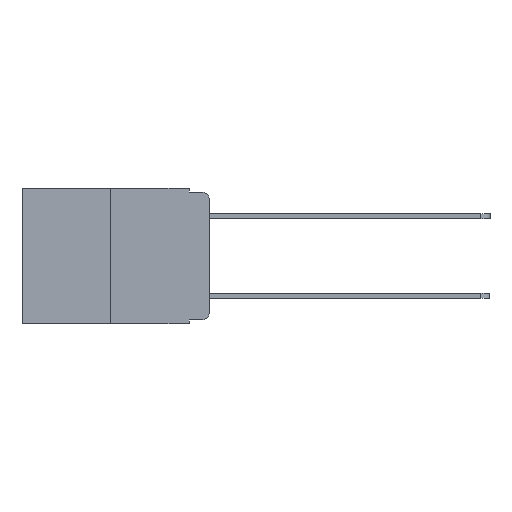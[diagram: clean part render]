
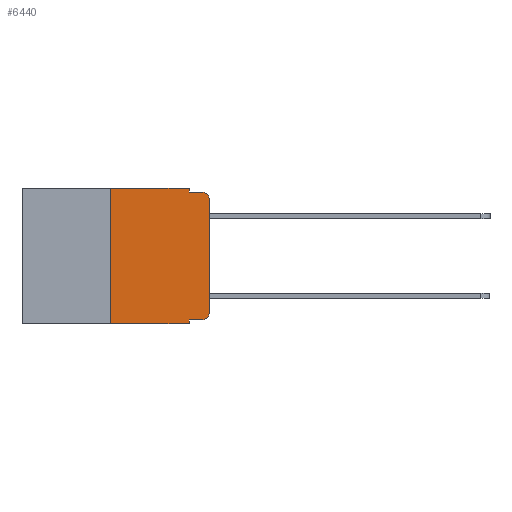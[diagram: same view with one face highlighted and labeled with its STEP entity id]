
A CAD part, left-side view. The second image highlights one B-rep face of the part: STEP entity #6440.
In plain terms, the highlighted planar face has unit normal (-1, 0, 0).
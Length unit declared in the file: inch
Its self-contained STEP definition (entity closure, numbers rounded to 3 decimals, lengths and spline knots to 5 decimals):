
#75 = VERTEX_POINT ( 'NONE', #7798 ) ;
#300 = CARTESIAN_POINT ( 'NONE',  ( 0., 0.02, -0.03 ) ) ;
#332 = EDGE_CURVE ( 'NONE', #7815, #8285, #4968, .T. ) ;
#638 = CARTESIAN_POINT ( 'NONE',  ( 0., 0.25, 0. ) ) ;
#748 = VERTEX_POINT ( 'NONE', #6219 ) ;
#782 = CARTESIAN_POINT ( 'NONE',  ( 0., 0.051, 0. ) ) ;
#843 = CARTESIAN_POINT ( 'NONE',  ( 0., 0.051, -0.333 ) ) ;
#997 = EDGE_CURVE ( 'NONE', #4513, #5603, #5073, .T. ) ;
#1048 = DIRECTION ( 'NONE',  ( -1., 0., 0. ) ) ;
#1443 = DIRECTION ( 'NONE',  ( 0., -1., 0. ) ) ;
#1632 = CARTESIAN_POINT ( 'NONE',  ( 0., 0., 0. ) ) ;
#1681 = CARTESIAN_POINT ( 'NONE',  ( 0., 0.051, 0. ) ) ;
#1826 = ORIENTED_EDGE ( 'NONE', *, *, #6490, .F. ) ;
#2148 = CARTESIAN_POINT ( 'NONE',  ( 0., 0.02, -0.313 ) ) ;
#2319 = ORIENTED_EDGE ( 'NONE', *, *, #8658, .T. ) ;
#2389 = LINE ( 'NONE', #1632, #7743 ) ;
#2480 = VECTOR ( 'NONE', #6686, 39.37008 ) ;
#2529 = ORIENTED_EDGE ( 'NONE', *, *, #10711, .F. ) ;
#2551 = CARTESIAN_POINT ( 'NONE',  ( 0., 0.051, -0.343 ) ) ;
#2722 = DIRECTION ( 'NONE',  ( 0., 0., 1. ) ) ;
#2818 = VECTOR ( 'NONE', #6099, 39.37008 ) ;
#2849 = ORIENTED_EDGE ( 'NONE', *, *, #9402, .F. ) ;
#2939 = LINE ( 'NONE', #3443, #7371 ) ;
#3002 = AXIS2_PLACEMENT_3D ( 'NONE', #10158, #3474, #5413 ) ;
#3008 = DIRECTION ( 'NONE',  ( 0., 0., -1. ) ) ;
#3443 = CARTESIAN_POINT ( 'NONE',  ( 0., 0.25, 0. ) ) ;
#3474 = DIRECTION ( 'NONE',  ( 1., 0., 0. ) ) ;
#3581 = CARTESIAN_POINT ( 'NONE',  ( 0., 0.051, -0.01 ) ) ;
#3630 = EDGE_CURVE ( 'NONE', #748, #8343, #2389, .T. ) ;
#3754 = PLANE ( 'NONE',  #3002 ) ;
#3837 = ORIENTED_EDGE ( 'NONE', *, *, #997, .F. ) ;
#4122 = DIRECTION ( 'NONE',  ( 0., 0., -1. ) ) ;
#4192 = CARTESIAN_POINT ( 'NONE',  ( 0., 0.02, -0.333 ) ) ;
#4513 = VERTEX_POINT ( 'NONE', #638 ) ;
#4563 = LINE ( 'NONE', #1681, #6491 ) ;
#4564 = EDGE_CURVE ( 'NONE', #75, #8273, #9414, .T. ) ;
#4637 = CARTESIAN_POINT ( 'NONE',  ( 0., 0.473, -0.343 ) ) ;
#4782 = CARTESIAN_POINT ( 'NONE',  ( 0., 0.473, 0. ) ) ;
#4785 = ORIENTED_EDGE ( 'NONE', *, *, #3630, .T. ) ;
#4827 = VECTOR ( 'NONE', #5310, 39.37008 ) ;
#4968 = LINE ( 'NONE', #4637, #2480 ) ;
#5039 = EDGE_CURVE ( 'NONE', #8343, #6675, #6914, .T. ) ;
#5073 = LINE ( 'NONE', #4782, #4827 ) ;
#5251 = VECTOR ( 'NONE', #1443, 39.37008 ) ;
#5298 = LINE ( 'NONE', #3581, #2818 ) ;
#5310 = DIRECTION ( 'NONE',  ( 0., -1., 0. ) ) ;
#5413 = DIRECTION ( 'NONE',  ( 0., 0., -1. ) ) ;
#5448 = ORIENTED_EDGE ( 'NONE', *, *, #4564, .T. ) ;
#5603 = VERTEX_POINT ( 'NONE', #5694 ) ;
#5694 = CARTESIAN_POINT ( 'NONE',  ( 0., 0.051, 0. ) ) ;
#5963 = AXIS2_PLACEMENT_3D ( 'NONE', #300, #1048, #4122 ) ;
#6099 = DIRECTION ( 'NONE',  ( 0., -1., 0. ) ) ;
#6168 = CARTESIAN_POINT ( 'NONE',  ( 0., 0.051, -0.01 ) ) ;
#6219 = CARTESIAN_POINT ( 'NONE',  ( 0., 0., -0.313 ) ) ;
#6440 = ADVANCED_FACE ( 'NONE', ( #9237 ), #3754, .F. ) ;
#6490 = EDGE_CURVE ( 'NONE', #5603, #10779, #4563, .T. ) ;
#6491 = VECTOR ( 'NONE', #8809, 39.37008 ) ;
#6675 = VERTEX_POINT ( 'NONE', #9421 ) ;
#6686 = DIRECTION ( 'NONE',  ( 0., -1., 0. ) ) ;
#6914 = CIRCLE ( 'NONE', #5963, 0.02 ) ;
#7137 = AXIS2_PLACEMENT_3D ( 'NONE', #2148, #7999, #3008 ) ;
#7371 = VECTOR ( 'NONE', #9264, 39.37008 ) ;
#7509 = DIRECTION ( 'NONE',  ( 0., 0., -1. ) ) ;
#7743 = VECTOR ( 'NONE', #2722, 39.37008 ) ;
#7798 = CARTESIAN_POINT ( 'NONE',  ( 0., 0.051, -0.333 ) ) ;
#7815 = VERTEX_POINT ( 'NONE', #8402 ) ;
#7999 = DIRECTION ( 'NONE',  ( -1., 0., 0. ) ) ;
#8120 = EDGE_LOOP ( 'NONE', ( #4785, #9952, #2529, #1826, #3837, #8952, #8730, #2849, #5448, #2319 ) ) ;
#8186 = VECTOR ( 'NONE', #7509, 39.37008 ) ;
#8273 = VERTEX_POINT ( 'NONE', #4192 ) ;
#8285 = VERTEX_POINT ( 'NONE', #2551 ) ;
#8343 = VERTEX_POINT ( 'NONE', #8469 ) ;
#8402 = CARTESIAN_POINT ( 'NONE',  ( 0., 0.25, -0.343 ) ) ;
#8469 = CARTESIAN_POINT ( 'NONE',  ( 0., 0., -0.03 ) ) ;
#8658 = EDGE_CURVE ( 'NONE', #8273, #748, #10463, .T. ) ;
#8730 = ORIENTED_EDGE ( 'NONE', *, *, #332, .T. ) ;
#8809 = DIRECTION ( 'NONE',  ( 0., 0., -1. ) ) ;
#8943 = EDGE_CURVE ( 'NONE', #7815, #4513, #2939, .T. ) ;
#8952 = ORIENTED_EDGE ( 'NONE', *, *, #8943, .F. ) ;
#9237 = FACE_OUTER_BOUND ( 'NONE', #8120, .T. ) ;
#9264 = DIRECTION ( 'NONE',  ( 0., 0., 1. ) ) ;
#9402 = EDGE_CURVE ( 'NONE', #75, #8285, #10358, .T. ) ;
#9414 = LINE ( 'NONE', #843, #5251 ) ;
#9421 = CARTESIAN_POINT ( 'NONE',  ( 0., 0.02, -0.01 ) ) ;
#9952 = ORIENTED_EDGE ( 'NONE', *, *, #5039, .T. ) ;
#10158 = CARTESIAN_POINT ( 'NONE',  ( 0., 0.473, 0. ) ) ;
#10358 = LINE ( 'NONE', #782, #8186 ) ;
#10463 = CIRCLE ( 'NONE', #7137, 0.02 ) ;
#10711 = EDGE_CURVE ( 'NONE', #10779, #6675, #5298, .T. ) ;
#10779 = VERTEX_POINT ( 'NONE', #6168 ) ;
